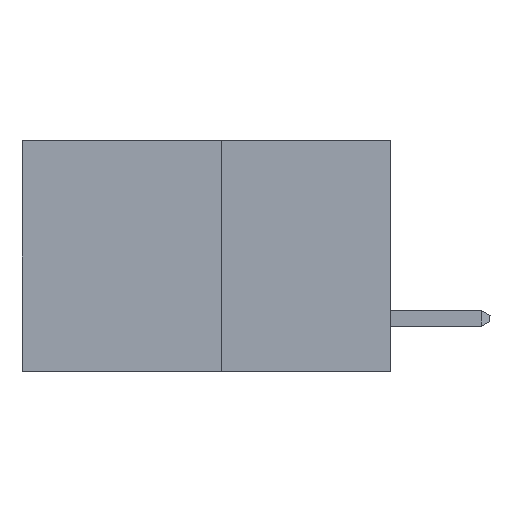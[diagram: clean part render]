
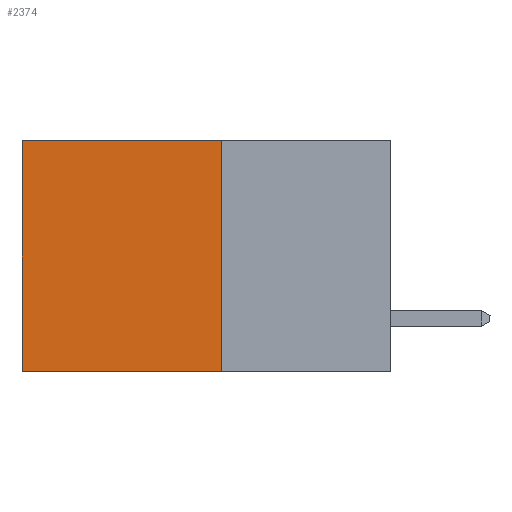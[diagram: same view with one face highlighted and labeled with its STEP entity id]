
A CAD part, left-side view. The second image highlights one B-rep face of the part: STEP entity #2374.
In plain terms, the highlighted planar face has unit normal (-1, 0, 0).
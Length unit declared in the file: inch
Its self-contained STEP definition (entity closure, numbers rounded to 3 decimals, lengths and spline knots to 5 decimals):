
#41 = DIRECTION ( 'NONE',  ( 0., 0., -1. ) ) ;
#240 = EDGE_CURVE ( 'NONE', #9173, #1354, #6622, .T. ) ;
#657 = VERTEX_POINT ( 'NONE', #6467 ) ;
#1354 = VERTEX_POINT ( 'NONE', #8118 ) ;
#1488 = AXIS2_PLACEMENT_3D ( 'NONE', #3325, #5671, #41 ) ;
#2017 = CARTESIAN_POINT ( 'NONE',  ( 0.277, 0.27, -0.37 ) ) ;
#2374 = ADVANCED_FACE ( 'NONE', ( #6139 ), #5691, .F. ) ;
#2754 = EDGE_CURVE ( 'NONE', #7918, #1354, #5151, .T. ) ;
#2800 = VECTOR ( 'NONE', #7377, 39.37008 ) ;
#3100 = ORIENTED_EDGE ( 'NONE', *, *, #240, .T. ) ;
#3149 = ORIENTED_EDGE ( 'NONE', *, *, #2754, .F. ) ;
#3227 = ORIENTED_EDGE ( 'NONE', *, *, #4186, .F. ) ;
#3243 = ORIENTED_EDGE ( 'NONE', *, *, #4984, .T. ) ;
#3325 = CARTESIAN_POINT ( 'NONE',  ( 0.277, 0.27, -0.37 ) ) ;
#3402 = VECTOR ( 'NONE', #8967, 39.37008 ) ;
#4186 = EDGE_CURVE ( 'NONE', #657, #7918, #7467, .T. ) ;
#4984 = EDGE_CURVE ( 'NONE', #657, #9173, #6627, .T. ) ;
#5151 = LINE ( 'NONE', #8848, #5360 ) ;
#5360 = VECTOR ( 'NONE', #7711, 39.37008 ) ;
#5671 = DIRECTION ( 'NONE',  ( 1., 0., 0. ) ) ;
#5691 = PLANE ( 'NONE',  #1488 ) ;
#6139 = FACE_OUTER_BOUND ( 'NONE', #9257, .T. ) ;
#6467 = CARTESIAN_POINT ( 'NONE',  ( 0.277, 0.27, 0. ) ) ;
#6622 = LINE ( 'NONE', #9006, #3402 ) ;
#6627 = LINE ( 'NONE', #7336, #2800 ) ;
#7263 = VECTOR ( 'NONE', #8222, 39.37008 ) ;
#7336 = CARTESIAN_POINT ( 'NONE',  ( 0.277, 0.27, 0. ) ) ;
#7377 = DIRECTION ( 'NONE',  ( 0., 1., 0. ) ) ;
#7467 = LINE ( 'NONE', #8703, #7263 ) ;
#7711 = DIRECTION ( 'NONE',  ( 0., 1., 0. ) ) ;
#7790 = CARTESIAN_POINT ( 'NONE',  ( 0.277, 0.59, 0. ) ) ;
#7918 = VERTEX_POINT ( 'NONE', #2017 ) ;
#8118 = CARTESIAN_POINT ( 'NONE',  ( 0.277, 0.59, -0.37 ) ) ;
#8222 = DIRECTION ( 'NONE',  ( 0., 0., -1. ) ) ;
#8703 = CARTESIAN_POINT ( 'NONE',  ( 0.277, 0.27, -0.37 ) ) ;
#8848 = CARTESIAN_POINT ( 'NONE',  ( 0.277, 0.27, -0.37 ) ) ;
#8967 = DIRECTION ( 'NONE',  ( 0., 0., -1. ) ) ;
#9006 = CARTESIAN_POINT ( 'NONE',  ( 0.277, 0.59, -0.37 ) ) ;
#9173 = VERTEX_POINT ( 'NONE', #7790 ) ;
#9257 = EDGE_LOOP ( 'NONE', ( #3100, #3149, #3227, #3243 ) ) ;
